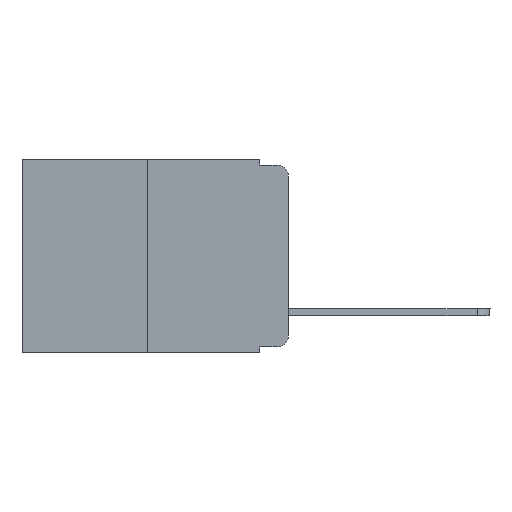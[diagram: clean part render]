
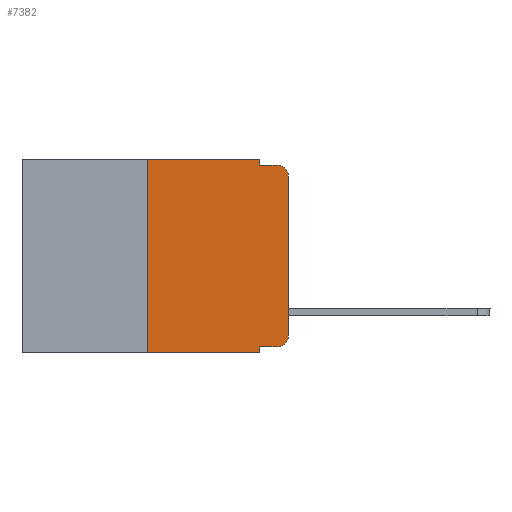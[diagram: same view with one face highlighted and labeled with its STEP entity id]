
A CAD part, left-side view. The second image highlights one B-rep face of the part: STEP entity #7382.
In plain terms, the highlighted planar face has unit normal (-1, 0, 0).
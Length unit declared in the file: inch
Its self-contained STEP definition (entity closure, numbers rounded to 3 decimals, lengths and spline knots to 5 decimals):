
#156 = CARTESIAN_POINT ( 'NONE',  ( 0., 0.473, -0.343 ) ) ;
#297 = LINE ( 'NONE', #13441, #11750 ) ;
#308 = VERTEX_POINT ( 'NONE', #6624 ) ;
#331 = CARTESIAN_POINT ( 'NONE',  ( 0., 0.25, 0. ) ) ;
#401 = CARTESIAN_POINT ( 'NONE',  ( 0., 0.473, 0. ) ) ;
#512 = DIRECTION ( 'NONE',  ( 0., -1., 0. ) ) ;
#594 = ORIENTED_EDGE ( 'NONE', *, *, #9620, .T. ) ;
#624 = LINE ( 'NONE', #4609, #13271 ) ;
#773 = CIRCLE ( 'NONE', #6127, 0.02 ) ;
#953 = VERTEX_POINT ( 'NONE', #6378 ) ;
#1073 = VECTOR ( 'NONE', #12231, 39.37008 ) ;
#1191 = EDGE_CURVE ( 'NONE', #13965, #10023, #3441, .T. ) ;
#1442 = ORIENTED_EDGE ( 'NONE', *, *, #1191, .T. ) ;
#1604 = CARTESIAN_POINT ( 'NONE',  ( 0., 0.02, -0.313 ) ) ;
#1919 = CARTESIAN_POINT ( 'NONE',  ( 0., 0.25, -0.343 ) ) ;
#2234 = ORIENTED_EDGE ( 'NONE', *, *, #4223, .T. ) ;
#2461 = EDGE_CURVE ( 'NONE', #8311, #4576, #13661, .T. ) ;
#3082 = CARTESIAN_POINT ( 'NONE',  ( 0., 0.051, -0.01 ) ) ;
#3441 = LINE ( 'NONE', #4907, #8299 ) ;
#3624 = DIRECTION ( 'NONE',  ( 0., 0., -1. ) ) ;
#3658 = EDGE_CURVE ( 'NONE', #13965, #953, #624, .T. ) ;
#3671 = CARTESIAN_POINT ( 'NONE',  ( 0., 0.25, 0. ) ) ;
#3755 = DIRECTION ( 'NONE',  ( 0., -1., 0. ) ) ;
#3953 = VERTEX_POINT ( 'NONE', #1919 ) ;
#4223 = EDGE_CURVE ( 'NONE', #6856, #6580, #773, .T. ) ;
#4248 = EDGE_CURVE ( 'NONE', #10023, #308, #10115, .T. ) ;
#4385 = LINE ( 'NONE', #156, #1073 ) ;
#4407 = VERTEX_POINT ( 'NONE', #3082 ) ;
#4576 = VERTEX_POINT ( 'NONE', #10075 ) ;
#4609 = CARTESIAN_POINT ( 'NONE',  ( 0., 0.051, 0. ) ) ;
#4655 = DIRECTION ( 'NONE',  ( 0., 0., -1. ) ) ;
#4907 = CARTESIAN_POINT ( 'NONE',  ( 0., 0.051, -0.333 ) ) ;
#5239 = DIRECTION ( 'NONE',  ( 0., 0., -1. ) ) ;
#5526 = CARTESIAN_POINT ( 'NONE',  ( 0., 0., -0.03 ) ) ;
#5579 = ORIENTED_EDGE ( 'NONE', *, *, #8837, .F. ) ;
#6069 = CARTESIAN_POINT ( 'NONE',  ( 0., 0.051, -0.01 ) ) ;
#6127 = AXIS2_PLACEMENT_3D ( 'NONE', #10912, #12950, #5239 ) ;
#6378 = CARTESIAN_POINT ( 'NONE',  ( 0., 0.051, -0.343 ) ) ;
#6580 = VERTEX_POINT ( 'NONE', #11050 ) ;
#6624 = CARTESIAN_POINT ( 'NONE',  ( 0., 0., -0.313 ) ) ;
#6665 = CARTESIAN_POINT ( 'NONE',  ( 0., 0.473, 0. ) ) ;
#6856 = VERTEX_POINT ( 'NONE', #5526 ) ;
#7032 = DIRECTION ( 'NONE',  ( -1., 0., 0. ) ) ;
#7154 = EDGE_CURVE ( 'NONE', #4407, #6580, #12320, .T. ) ;
#7367 = VECTOR ( 'NONE', #7708, 39.37008 ) ;
#7382 = ADVANCED_FACE ( 'NONE', ( #12643 ), #11048, .F. ) ;
#7572 = AXIS2_PLACEMENT_3D ( 'NONE', #1604, #7032, #3624 ) ;
#7691 = ORIENTED_EDGE ( 'NONE', *, *, #7154, .F. ) ;
#7708 = DIRECTION ( 'NONE',  ( 0., 0., 1. ) ) ;
#8299 = VECTOR ( 'NONE', #512, 39.37008 ) ;
#8311 = VERTEX_POINT ( 'NONE', #3671 ) ;
#8431 = LINE ( 'NONE', #13270, #7367 ) ;
#8557 = ORIENTED_EDGE ( 'NONE', *, *, #3658, .F. ) ;
#8837 = EDGE_CURVE ( 'NONE', #3953, #8311, #13854, .T. ) ;
#8953 = ORIENTED_EDGE ( 'NONE', *, *, #10253, .F. ) ;
#9068 = EDGE_LOOP ( 'NONE', ( #594, #2234, #7691, #8953, #10206, #5579, #9725, #8557, #1442, #11203 ) ) ;
#9167 = DIRECTION ( 'NONE',  ( 0., 0., 1. ) ) ;
#9476 = VECTOR ( 'NONE', #9167, 39.37008 ) ;
#9620 = EDGE_CURVE ( 'NONE', #308, #6856, #8431, .T. ) ;
#9725 = ORIENTED_EDGE ( 'NONE', *, *, #12470, .T. ) ;
#10023 = VERTEX_POINT ( 'NONE', #10649 ) ;
#10075 = CARTESIAN_POINT ( 'NONE',  ( 0., 0.051, 0. ) ) ;
#10115 = CIRCLE ( 'NONE', #7572, 0.02 ) ;
#10206 = ORIENTED_EDGE ( 'NONE', *, *, #2461, .F. ) ;
#10253 = EDGE_CURVE ( 'NONE', #4576, #4407, #297, .T. ) ;
#10649 = CARTESIAN_POINT ( 'NONE',  ( 0., 0.02, -0.333 ) ) ;
#10912 = CARTESIAN_POINT ( 'NONE',  ( 0., 0.02, -0.03 ) ) ;
#11048 = PLANE ( 'NONE',  #14359 ) ;
#11050 = CARTESIAN_POINT ( 'NONE',  ( 0., 0.02, -0.01 ) ) ;
#11203 = ORIENTED_EDGE ( 'NONE', *, *, #4248, .T. ) ;
#11255 = DIRECTION ( 'NONE',  ( 0., 0., -1. ) ) ;
#11750 = VECTOR ( 'NONE', #11255, 39.37008 ) ;
#12145 = VECTOR ( 'NONE', #3755, 39.37008 ) ;
#12231 = DIRECTION ( 'NONE',  ( 0., -1., 0. ) ) ;
#12320 = LINE ( 'NONE', #6069, #12145 ) ;
#12470 = EDGE_CURVE ( 'NONE', #3953, #953, #4385, .T. ) ;
#12616 = CARTESIAN_POINT ( 'NONE',  ( 0., 0.051, -0.333 ) ) ;
#12643 = FACE_OUTER_BOUND ( 'NONE', #9068, .T. ) ;
#12738 = DIRECTION ( 'NONE',  ( 0., -1., 0. ) ) ;
#12950 = DIRECTION ( 'NONE',  ( -1., 0., 0. ) ) ;
#12957 = VECTOR ( 'NONE', #12738, 39.37008 ) ;
#13182 = DIRECTION ( 'NONE',  ( 0., 0., -1. ) ) ;
#13270 = CARTESIAN_POINT ( 'NONE',  ( 0., 0., 0. ) ) ;
#13271 = VECTOR ( 'NONE', #4655, 39.37008 ) ;
#13281 = DIRECTION ( 'NONE',  ( 1., 0., 0. ) ) ;
#13441 = CARTESIAN_POINT ( 'NONE',  ( 0., 0.051, 0. ) ) ;
#13661 = LINE ( 'NONE', #401, #12957 ) ;
#13854 = LINE ( 'NONE', #331, #9476 ) ;
#13965 = VERTEX_POINT ( 'NONE', #12616 ) ;
#14359 = AXIS2_PLACEMENT_3D ( 'NONE', #6665, #13281, #13182 ) ;
